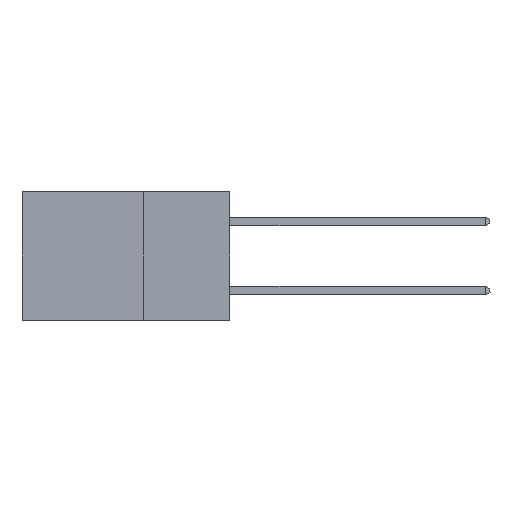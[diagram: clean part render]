
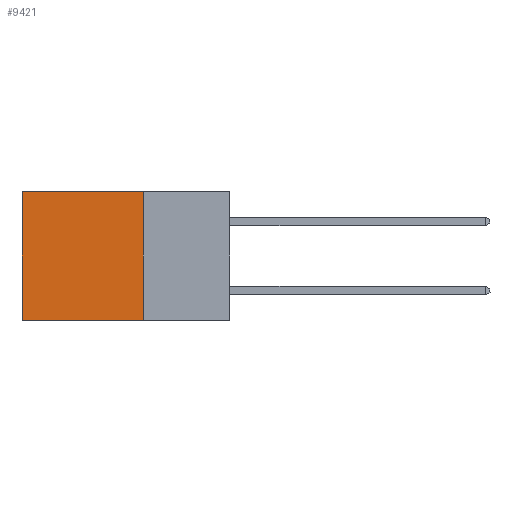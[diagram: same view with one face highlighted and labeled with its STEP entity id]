
A CAD part, left-side view. The second image highlights one B-rep face of the part: STEP entity #9421.
In plain terms, the highlighted planar face has unit normal (-1, 0, 0).
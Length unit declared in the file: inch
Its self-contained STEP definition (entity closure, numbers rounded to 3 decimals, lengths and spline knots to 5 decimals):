
#193 = LINE ( 'NONE', #2498, #20864 ) ;
#530 = CARTESIAN_POINT ( 'NONE',  ( 0.298, 0.25, 0. ) ) ;
#1509 = LINE ( 'NONE', #10703, #4630 ) ;
#1727 = CARTESIAN_POINT ( 'NONE',  ( 0.298, 0.6, 0. ) ) ;
#2498 = CARTESIAN_POINT ( 'NONE',  ( 0.298, 0.25, -0.37 ) ) ;
#2617 = ORIENTED_EDGE ( 'NONE', *, *, #21805, .T. ) ;
#4010 = CARTESIAN_POINT ( 'NONE',  ( 0.298, 0.6, -0.37 ) ) ;
#4630 = VECTOR ( 'NONE', #12558, 39.37008 ) ;
#4702 = EDGE_LOOP ( 'NONE', ( #2617, #6807, #19866, #13783 ) ) ;
#5784 = DIRECTION ( 'NONE',  ( 0., 0., -1. ) ) ;
#5874 = CARTESIAN_POINT ( 'NONE',  ( 0.298, 0.25, 0. ) ) ;
#6030 = FACE_OUTER_BOUND ( 'NONE', #4702, .T. ) ;
#6031 = LINE ( 'NONE', #5874, #8882 ) ;
#6204 = DIRECTION ( 'NONE',  ( 0., 1., 0. ) ) ;
#6807 = ORIENTED_EDGE ( 'NONE', *, *, #8059, .F. ) ;
#8059 = EDGE_CURVE ( 'NONE', #18931, #10338, #193, .T. ) ;
#8384 = DIRECTION ( 'NONE',  ( 1., 0., 0. ) ) ;
#8882 = VECTOR ( 'NONE', #5784, 39.37008 ) ;
#9421 = ADVANCED_FACE ( 'NONE', ( #6030 ), #9999, .F. ) ;
#9999 = PLANE ( 'NONE',  #20759 ) ;
#10338 = VERTEX_POINT ( 'NONE', #4010 ) ;
#10703 = CARTESIAN_POINT ( 'NONE',  ( 0.298, 0.6, 0. ) ) ;
#11645 = LINE ( 'NONE', #530, #17866 ) ;
#12558 = DIRECTION ( 'NONE',  ( 0., 0., -1. ) ) ;
#13654 = VERTEX_POINT ( 'NONE', #20438 ) ;
#13770 = DIRECTION ( 'NONE',  ( 0., 0., -1. ) ) ;
#13783 = ORIENTED_EDGE ( 'NONE', *, *, #20576, .T. ) ;
#16677 = DIRECTION ( 'NONE',  ( 0., 1., 0. ) ) ;
#16714 = CARTESIAN_POINT ( 'NONE',  ( 0.298, 0.25, -0.37 ) ) ;
#17866 = VECTOR ( 'NONE', #6204, 39.37008 ) ;
#18931 = VERTEX_POINT ( 'NONE', #16714 ) ;
#19209 = VERTEX_POINT ( 'NONE', #1727 ) ;
#19866 = ORIENTED_EDGE ( 'NONE', *, *, #25598, .F. ) ;
#20438 = CARTESIAN_POINT ( 'NONE',  ( 0.298, 0.25, 0. ) ) ;
#20576 = EDGE_CURVE ( 'NONE', #13654, #19209, #11645, .T. ) ;
#20759 = AXIS2_PLACEMENT_3D ( 'NONE', #25896, #8384, #13770 ) ;
#20864 = VECTOR ( 'NONE', #16677, 39.37008 ) ;
#21805 = EDGE_CURVE ( 'NONE', #19209, #10338, #1509, .T. ) ;
#25598 = EDGE_CURVE ( 'NONE', #13654, #18931, #6031, .T. ) ;
#25896 = CARTESIAN_POINT ( 'NONE',  ( 0.298, 0.25, 0. ) ) ;
